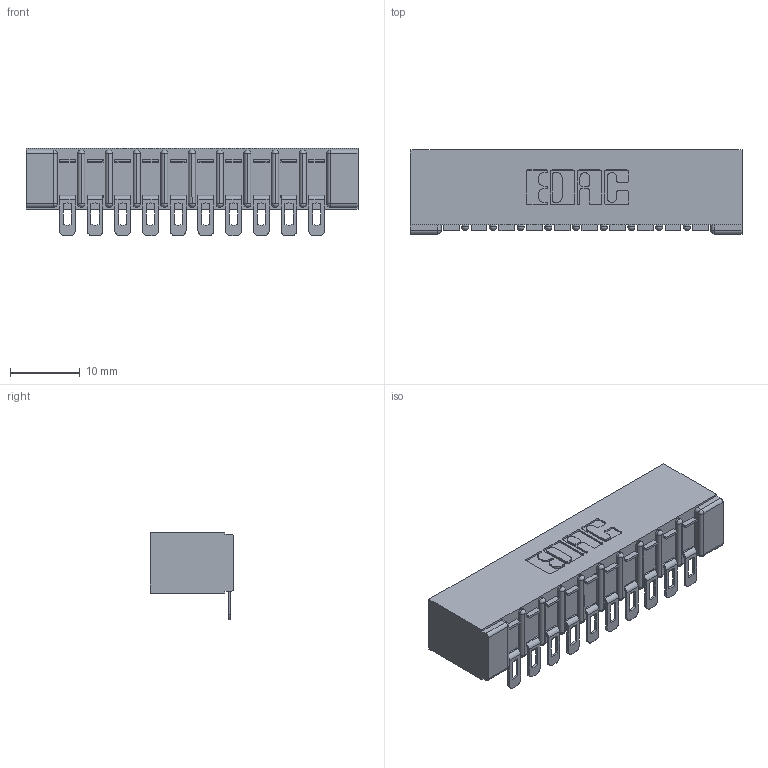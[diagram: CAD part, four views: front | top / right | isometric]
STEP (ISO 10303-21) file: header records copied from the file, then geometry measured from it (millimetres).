
FILE_DESCRIPTION (( 'STEP AP203' ), '1' );
FILE_NAME ('307-010-554-101.STEP', '2018-08-02T21:26:50', ( '' ), ( '' ), 'SwSTEP 2.0', 'SolidWorks 2016', '' );
FILE_SCHEMA (( 'CONFIG_CONTROL_DESIGN' ));
Length unit declared in the file: inch
Products named in the file (3): 307 Part_No Mounting Lugs; 307-290-002_554; 307-010-554-101
Assembly tree (11 placements, depth 2):
  307-010-554-101
    307 Part_No Mounting Lugs
    307-290-002_554  x10
Bounding box: 47.5 x 12.01 x 12.52 mm (x, y, z)
Volume: 3375.4 mm3; surface area: 6020.3 mm2
Topology: 11 solids, 11 shells, 931 faces, 2829 edges, 1854 vertices
Faces by surface type: plane 526, cylinder 383, sphere 22
Entity records: 13205 total; most frequent: CARTESIAN_POINT 2222, ORIENTED_EDGE 2212, DIRECTION 2178, EDGE_CURVE 1106, LINE 826, VECTOR 826, VERTEX_POINT 720, AXIS2_PLACEMENT_3D 676
